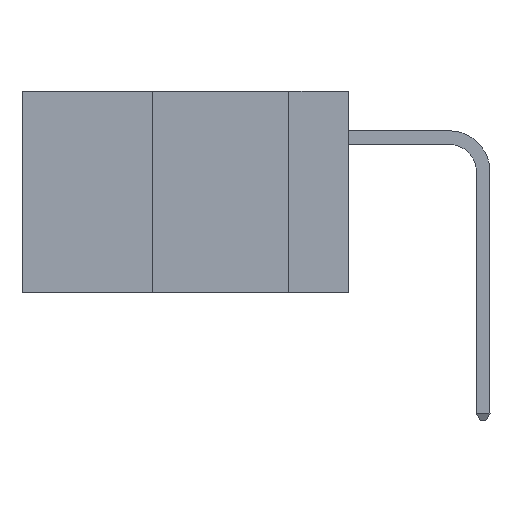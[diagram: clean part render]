
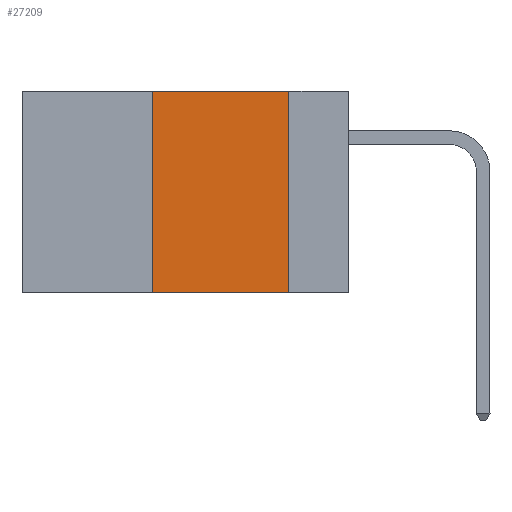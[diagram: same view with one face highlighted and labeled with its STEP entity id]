
A CAD part, left-side view. The second image highlights one B-rep face of the part: STEP entity #27209.
In plain terms, the highlighted planar face has unit normal (-1, 0, 0).
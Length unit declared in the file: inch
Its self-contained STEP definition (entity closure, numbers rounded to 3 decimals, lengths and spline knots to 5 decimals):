
#672 = CARTESIAN_POINT ( 'NONE',  ( 0., 0.36, -0.37 ) ) ;
#1599 = ORIENTED_EDGE ( 'NONE', *, *, #5823, .T. ) ;
#1686 = DIRECTION ( 'NONE',  ( 0., -1., 0. ) ) ;
#1788 = AXIS2_PLACEMENT_3D ( 'NONE', #26859, #14700, #6703 ) ;
#2159 = LINE ( 'NONE', #26181, #18114 ) ;
#2736 = CARTESIAN_POINT ( 'NONE',  ( 0., 0.6, -0.37 ) ) ;
#3655 = VECTOR ( 'NONE', #24524, 39.37008 ) ;
#4312 = DIRECTION ( 'NONE',  ( 0., 0., -1. ) ) ;
#4703 = ORIENTED_EDGE ( 'NONE', *, *, #8246, .F. ) ;
#5787 = VERTEX_POINT ( 'NONE', #672 ) ;
#5823 = EDGE_CURVE ( 'NONE', #5787, #29001, #7397, .T. ) ;
#6476 = ORIENTED_EDGE ( 'NONE', *, *, #20957, .F. ) ;
#6693 = VECTOR ( 'NONE', #22009, 39.37008 ) ;
#6703 = DIRECTION ( 'NONE',  ( 0., 0., -1. ) ) ;
#7397 = LINE ( 'NONE', #2736, #3655 ) ;
#7428 = CARTESIAN_POINT ( 'NONE',  ( 0., 0.36, 0. ) ) ;
#8157 = CARTESIAN_POINT ( 'NONE',  ( 0., 0.11, 0. ) ) ;
#8246 = EDGE_CURVE ( 'NONE', #30736, #24005, #2159, .T. ) ;
#11928 = LINE ( 'NONE', #7428, #6693 ) ;
#14063 = EDGE_CURVE ( 'NONE', #24005, #29001, #31357, .T. ) ;
#14700 = DIRECTION ( 'NONE',  ( 1., 0., 0. ) ) ;
#16473 = PLANE ( 'NONE',  #1788 ) ;
#16655 = CARTESIAN_POINT ( 'NONE',  ( 0., 0.11, 0. ) ) ;
#17103 = FACE_OUTER_BOUND ( 'NONE', #18399, .T. ) ;
#18114 = VECTOR ( 'NONE', #1686, 39.37008 ) ;
#18399 = EDGE_LOOP ( 'NONE', ( #19463, #4703, #6476, #1599 ) ) ;
#18621 = VECTOR ( 'NONE', #4312, 39.37008 ) ;
#19463 = ORIENTED_EDGE ( 'NONE', *, *, #14063, .F. ) ;
#20957 = EDGE_CURVE ( 'NONE', #5787, #30736, #11928, .T. ) ;
#22009 = DIRECTION ( 'NONE',  ( 0., 0., 1. ) ) ;
#22192 = CARTESIAN_POINT ( 'NONE',  ( 0., 0.36, 0. ) ) ;
#24005 = VERTEX_POINT ( 'NONE', #8157 ) ;
#24524 = DIRECTION ( 'NONE',  ( 0., -1., 0. ) ) ;
#26181 = CARTESIAN_POINT ( 'NONE',  ( 0., 0.6, 0. ) ) ;
#26859 = CARTESIAN_POINT ( 'NONE',  ( 0., 0.6, 0. ) ) ;
#27209 = ADVANCED_FACE ( 'NONE', ( #17103 ), #16473, .F. ) ;
#29001 = VERTEX_POINT ( 'NONE', #31462 ) ;
#30736 = VERTEX_POINT ( 'NONE', #22192 ) ;
#31357 = LINE ( 'NONE', #16655, #18621 ) ;
#31462 = CARTESIAN_POINT ( 'NONE',  ( 0., 0.11, -0.37 ) ) ;
